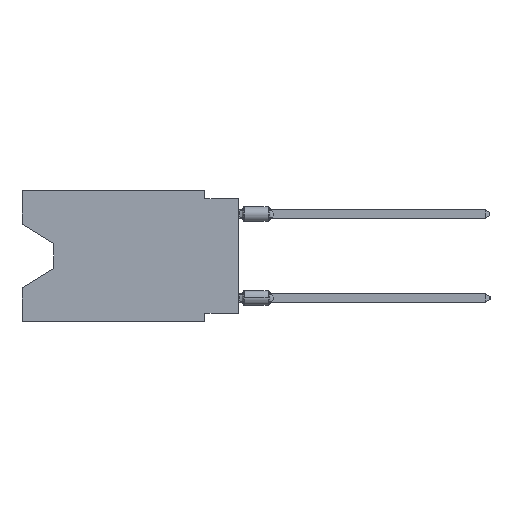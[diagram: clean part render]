
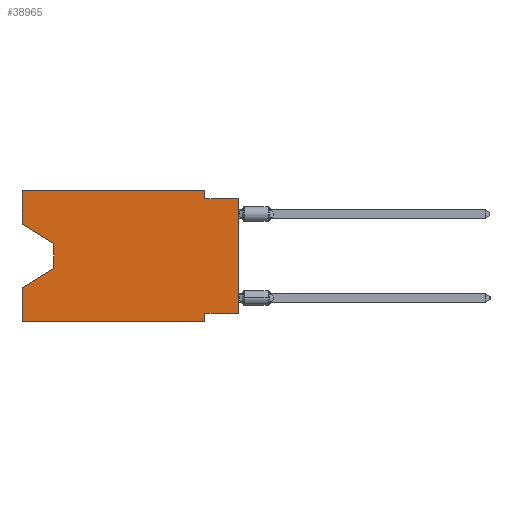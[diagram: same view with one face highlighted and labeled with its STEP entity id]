
A CAD part, left-side view. The second image highlights one B-rep face of the part: STEP entity #38965.
In plain terms, the highlighted planar face has unit normal (-1, 0, 0).
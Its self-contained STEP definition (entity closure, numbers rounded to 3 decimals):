
#468 = CARTESIAN_POINT ( 'NONE',  ( 0., 2.54, -9.906 ) ) ;
#530 = VECTOR ( 'NONE', #52656, 1000. ) ;
#773 = VECTOR ( 'NONE', #23028, 1000. ) ;
#1965 = CARTESIAN_POINT ( 'NONE',  ( 0., 13.97, -5.893 ) ) ;
#2276 = LINE ( 'NONE', #1965, #13945 ) ;
#2366 = CARTESIAN_POINT ( 'NONE',  ( 0., 16.383, 0. ) ) ;
#3361 = CARTESIAN_POINT ( 'NONE',  ( 0., 16.383, 0. ) ) ;
#3837 = EDGE_CURVE ( 'NONE', #42505, #63106, #15257, .T. ) ;
#3855 = CARTESIAN_POINT ( 'NONE',  ( 0., 0., -0.635 ) ) ;
#5777 = VERTEX_POINT ( 'NONE', #13210 ) ;
#6086 = DIRECTION ( 'NONE',  ( 0., -1., 0. ) ) ;
#6162 = EDGE_CURVE ( 'NONE', #18863, #5777, #23704, .T. ) ;
#6404 = LINE ( 'NONE', #55502, #60355 ) ;
#7250 = DIRECTION ( 'NONE',  ( 0., 0., -1. ) ) ;
#7912 = EDGE_CURVE ( 'NONE', #27970, #40399, #48475, .T. ) ;
#8192 = CARTESIAN_POINT ( 'NONE',  ( 0., 2.54, 0. ) ) ;
#8270 = LINE ( 'NONE', #27855, #773 ) ;
#10559 = EDGE_CURVE ( 'NONE', #26138, #37145, #17904, .T. ) ;
#11092 = DIRECTION ( 'NONE',  ( 0., 0., 1. ) ) ;
#11386 = VECTOR ( 'NONE', #21620, 1000. ) ;
#11468 = EDGE_CURVE ( 'NONE', #42505, #26138, #35320, .T. ) ;
#11500 = ORIENTED_EDGE ( 'NONE', *, *, #51850, .T. ) ;
#11586 = DIRECTION ( 'NONE',  ( 0., 0., 1. ) ) ;
#11772 = VERTEX_POINT ( 'NONE', #53550 ) ;
#11899 = LINE ( 'NONE', #46577, #23201 ) ;
#13210 = CARTESIAN_POINT ( 'NONE',  ( 0., 2.54, -9.271 ) ) ;
#13945 = VECTOR ( 'NONE', #41734, 1000. ) ;
#14353 = ORIENTED_EDGE ( 'NONE', *, *, #28824, .F. ) ;
#14577 = VECTOR ( 'NONE', #17956, 1000. ) ;
#15257 = LINE ( 'NONE', #54749, #49253 ) ;
#17364 = ORIENTED_EDGE ( 'NONE', *, *, #3837, .F. ) ;
#17554 = ORIENTED_EDGE ( 'NONE', *, *, #55713, .F. ) ;
#17904 = LINE ( 'NONE', #62502, #48782 ) ;
#17920 = ORIENTED_EDGE ( 'NONE', *, *, #25946, .T. ) ;
#17956 = DIRECTION ( 'NONE',  ( 0., 1., 0. ) ) ;
#18863 = VERTEX_POINT ( 'NONE', #57365 ) ;
#20632 = ORIENTED_EDGE ( 'NONE', *, *, #41028, .F. ) ;
#20998 = LINE ( 'NONE', #468, #32642 ) ;
#21620 = DIRECTION ( 'NONE',  ( 0., 0., -1. ) ) ;
#23028 = DIRECTION ( 'NONE',  ( 0., 0., 1. ) ) ;
#23201 = VECTOR ( 'NONE', #11586, 1000. ) ;
#23411 = DIRECTION ( 'NONE',  ( 0., -1., 0. ) ) ;
#23704 = LINE ( 'NONE', #62870, #14577 ) ;
#25192 = DIRECTION ( 'NONE',  ( 0., 0., -1. ) ) ;
#25946 = EDGE_CURVE ( 'NONE', #11772, #51590, #38518, .T. ) ;
#26138 = VERTEX_POINT ( 'NONE', #56133 ) ;
#27449 = FACE_OUTER_BOUND ( 'NONE', #36139, .T. ) ;
#27549 = DIRECTION ( 'NONE',  ( 0., 0., -1. ) ) ;
#27855 = CARTESIAN_POINT ( 'NONE',  ( 0., 16.383, 0. ) ) ;
#27970 = VERTEX_POINT ( 'NONE', #59742 ) ;
#28824 = EDGE_CURVE ( 'NONE', #11772, #43904, #8270, .T. ) ;
#31010 = ORIENTED_EDGE ( 'NONE', *, *, #10559, .T. ) ;
#32642 = VECTOR ( 'NONE', #25192, 1000. ) ;
#33550 = ORIENTED_EDGE ( 'NONE', *, *, #11468, .T. ) ;
#34310 = AXIS2_PLACEMENT_3D ( 'NONE', #3361, #51555, #7250 ) ;
#35320 = LINE ( 'NONE', #49437, #40669 ) ;
#35370 = VECTOR ( 'NONE', #23411, 1000. ) ;
#35419 = CARTESIAN_POINT ( 'NONE',  ( 0., 16.383, -7.36 ) ) ;
#36139 = EDGE_LOOP ( 'NONE', ( #33550, #31010, #11500, #14353, #17920, #20632, #48739, #50954, #53643, #17554, #42557, #17364 ) ) ;
#37145 = VERTEX_POINT ( 'NONE', #38188 ) ;
#38188 = CARTESIAN_POINT ( 'NONE',  ( 0., 13.97, -5.893 ) ) ;
#38518 = LINE ( 'NONE', #43635, #530 ) ;
#38965 = ADVANCED_FACE ( 'NONE', ( #27449 ), #41893, .F. ) ;
#40399 = VERTEX_POINT ( 'NONE', #41979 ) ;
#40669 = VECTOR ( 'NONE', #44282, 1000. ) ;
#40822 = VERTEX_POINT ( 'NONE', #8192 ) ;
#41028 = EDGE_CURVE ( 'NONE', #5777, #51590, #20998, .T. ) ;
#41201 = LINE ( 'NONE', #52664, #11386 ) ;
#41503 = EDGE_CURVE ( 'NONE', #63106, #40822, #6404, .T. ) ;
#41734 = DIRECTION ( 'NONE',  ( 0., 0.855, -0.519 ) ) ;
#41893 = PLANE ( 'NONE',  #34310 ) ;
#41979 = CARTESIAN_POINT ( 'NONE',  ( 0., 0., -0.635 ) ) ;
#42505 = VERTEX_POINT ( 'NONE', #42781 ) ;
#42557 = ORIENTED_EDGE ( 'NONE', *, *, #41503, .F. ) ;
#42781 = CARTESIAN_POINT ( 'NONE',  ( 0., 16.383, -2.546 ) ) ;
#43635 = CARTESIAN_POINT ( 'NONE',  ( 0., 16.383, -9.906 ) ) ;
#43904 = VERTEX_POINT ( 'NONE', #35419 ) ;
#44282 = DIRECTION ( 'NONE',  ( 0., -0.855, -0.519 ) ) ;
#46577 = CARTESIAN_POINT ( 'NONE',  ( 0., 0., 0. ) ) ;
#48475 = LINE ( 'NONE', #3855, #35370 ) ;
#48739 = ORIENTED_EDGE ( 'NONE', *, *, #6162, .F. ) ;
#48782 = VECTOR ( 'NONE', #27549, 1000. ) ;
#49253 = VECTOR ( 'NONE', #11092, 1000. ) ;
#49437 = CARTESIAN_POINT ( 'NONE',  ( 0., 16.383, -2.546 ) ) ;
#50954 = ORIENTED_EDGE ( 'NONE', *, *, #62373, .T. ) ;
#51555 = DIRECTION ( 'NONE',  ( 1., 0., 0. ) ) ;
#51590 = VERTEX_POINT ( 'NONE', #63271 ) ;
#51850 = EDGE_CURVE ( 'NONE', #37145, #43904, #2276, .T. ) ;
#52656 = DIRECTION ( 'NONE',  ( 0., -1., 0. ) ) ;
#52664 = CARTESIAN_POINT ( 'NONE',  ( 0., 2.54, 0. ) ) ;
#53550 = CARTESIAN_POINT ( 'NONE',  ( 0., 16.383, -9.906 ) ) ;
#53643 = ORIENTED_EDGE ( 'NONE', *, *, #7912, .F. ) ;
#54749 = CARTESIAN_POINT ( 'NONE',  ( 0., 16.383, 0. ) ) ;
#55502 = CARTESIAN_POINT ( 'NONE',  ( 0., 16.383, 0. ) ) ;
#55713 = EDGE_CURVE ( 'NONE', #40822, #27970, #41201, .T. ) ;
#56133 = CARTESIAN_POINT ( 'NONE',  ( 0., 13.97, -4.013 ) ) ;
#57365 = CARTESIAN_POINT ( 'NONE',  ( 0., 0., -9.271 ) ) ;
#59742 = CARTESIAN_POINT ( 'NONE',  ( 0., 2.54, -0.635 ) ) ;
#60355 = VECTOR ( 'NONE', #6086, 1000. ) ;
#62373 = EDGE_CURVE ( 'NONE', #18863, #40399, #11899, .T. ) ;
#62502 = CARTESIAN_POINT ( 'NONE',  ( 0., 13.97, -4.013 ) ) ;
#62870 = CARTESIAN_POINT ( 'NONE',  ( 0., 0., -9.271 ) ) ;
#63106 = VERTEX_POINT ( 'NONE', #2366 ) ;
#63271 = CARTESIAN_POINT ( 'NONE',  ( 0., 2.54, -9.906 ) ) ;
